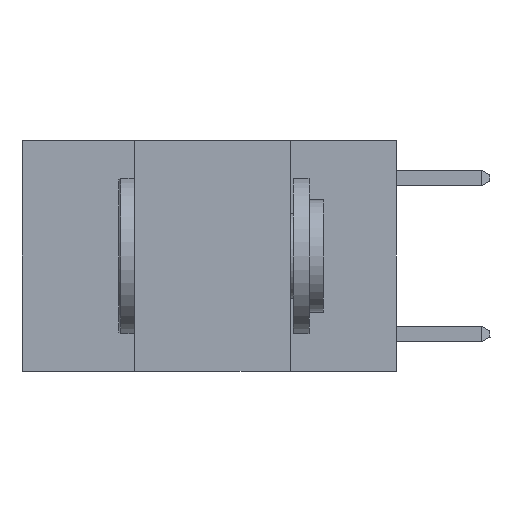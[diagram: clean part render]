
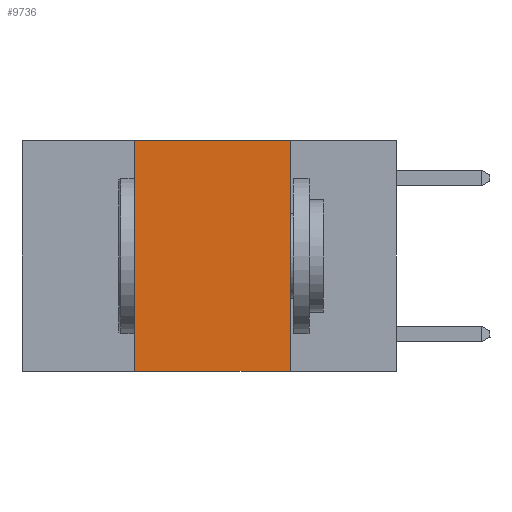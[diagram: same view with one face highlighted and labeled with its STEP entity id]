
A CAD part, left-side view. The second image highlights one B-rep face of the part: STEP entity #9736.
In plain terms, the highlighted planar face has unit normal (-1, 0, 0).
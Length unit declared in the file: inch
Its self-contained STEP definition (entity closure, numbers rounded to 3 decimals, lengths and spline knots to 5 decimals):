
#576 = LINE ( 'NONE', #6396, #11171 ) ;
#1180 = CARTESIAN_POINT ( 'NONE',  ( 0., 0.6, 0. ) ) ;
#2076 = DIRECTION ( 'NONE',  ( 0., -1., 0. ) ) ;
#2303 = LINE ( 'NONE', #8090, #14329 ) ;
#3095 = FACE_OUTER_BOUND ( 'NONE', #7483, .T. ) ;
#3254 = CARTESIAN_POINT ( 'NONE',  ( 0., 0.6, 0. ) ) ;
#3384 = EDGE_CURVE ( 'NONE', #13203, #10158, #2303, .T. ) ;
#3540 = CARTESIAN_POINT ( 'NONE',  ( 0., 0.17, 0. ) ) ;
#3759 = CARTESIAN_POINT ( 'NONE',  ( 0., 0.17, 0. ) ) ;
#3961 = EDGE_CURVE ( 'NONE', #4298, #10158, #13851, .T. ) ;
#4205 = CARTESIAN_POINT ( 'NONE',  ( 0., 0.17, -0.37 ) ) ;
#4298 = VERTEX_POINT ( 'NONE', #3540 ) ;
#4625 = ORIENTED_EDGE ( 'NONE', *, *, #11669, .F. ) ;
#4944 = CARTESIAN_POINT ( 'NONE',  ( 0., 0.42, 0. ) ) ;
#6396 = CARTESIAN_POINT ( 'NONE',  ( 0., 0.42, 0. ) ) ;
#6978 = DIRECTION ( 'NONE',  ( 0., 0., -1. ) ) ;
#7483 = EDGE_LOOP ( 'NONE', ( #14231, #4625, #12638, #14382 ) ) ;
#8090 = CARTESIAN_POINT ( 'NONE',  ( 0., 0.6, -0.37 ) ) ;
#9150 = EDGE_CURVE ( 'NONE', #13203, #9525, #576, .T. ) ;
#9525 = VERTEX_POINT ( 'NONE', #4944 ) ;
#9736 = ADVANCED_FACE ( 'NONE', ( #3095 ), #14409, .F. ) ;
#10133 = DIRECTION ( 'NONE',  ( 0., 0., -1. ) ) ;
#10158 = VERTEX_POINT ( 'NONE', #4205 ) ;
#11171 = VECTOR ( 'NONE', #11418, 39.37008 ) ;
#11418 = DIRECTION ( 'NONE',  ( 0., 0., 1. ) ) ;
#11568 = DIRECTION ( 'NONE',  ( 1., 0., 0. ) ) ;
#11669 = EDGE_CURVE ( 'NONE', #9525, #4298, #12115, .T. ) ;
#12115 = LINE ( 'NONE', #3254, #13387 ) ;
#12638 = ORIENTED_EDGE ( 'NONE', *, *, #9150, .F. ) ;
#13203 = VERTEX_POINT ( 'NONE', #13824 ) ;
#13387 = VECTOR ( 'NONE', #17734, 39.37008 ) ;
#13824 = CARTESIAN_POINT ( 'NONE',  ( 0., 0.42, -0.37 ) ) ;
#13851 = LINE ( 'NONE', #3759, #15616 ) ;
#14231 = ORIENTED_EDGE ( 'NONE', *, *, #3961, .F. ) ;
#14329 = VECTOR ( 'NONE', #2076, 39.37008 ) ;
#14382 = ORIENTED_EDGE ( 'NONE', *, *, #3384, .T. ) ;
#14409 = PLANE ( 'NONE',  #16688 ) ;
#15616 = VECTOR ( 'NONE', #6978, 39.37008 ) ;
#16688 = AXIS2_PLACEMENT_3D ( 'NONE', #1180, #11568, #10133 ) ;
#17734 = DIRECTION ( 'NONE',  ( 0., -1., 0. ) ) ;
